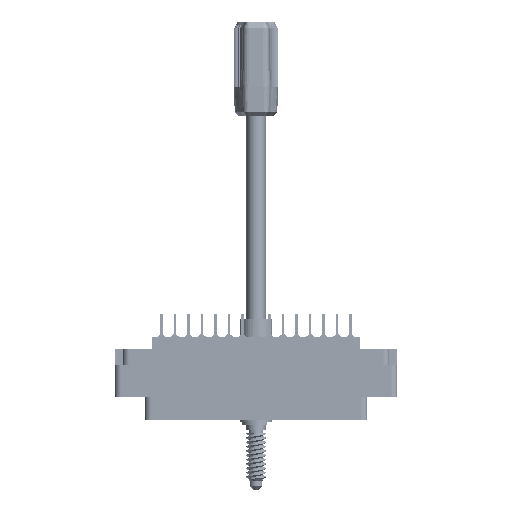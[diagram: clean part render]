
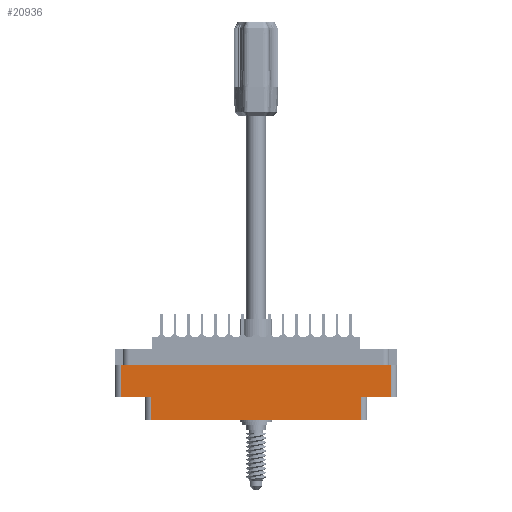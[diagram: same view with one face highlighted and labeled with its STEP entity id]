
A CAD part, front view. The second image highlights one B-rep face of the part: STEP entity #20936.
In plain terms, the highlighted planar face has unit normal (0, -1, 0).
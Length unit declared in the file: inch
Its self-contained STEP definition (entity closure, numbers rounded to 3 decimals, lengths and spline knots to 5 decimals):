
#2344 = LINE ( 'NONE', #57740, #59370 ) ;
#3108 = VERTEX_POINT ( 'NONE', #76428 ) ;
#3857 = CARTESIAN_POINT ( 'NONE',  ( -1.359, -0.617, -0.798 ) ) ;
#4095 = CARTESIAN_POINT ( 'NONE',  ( -1.297, -0.617, -0.578 ) ) ;
#4109 = ORIENTED_EDGE ( 'NONE', *, *, #5553, .F. ) ;
#5553 = EDGE_CURVE ( 'NONE', #71002, #6248, #46296, .T. ) ;
#6248 = VERTEX_POINT ( 'NONE', #72584 ) ;
#6738 = VERTEX_POINT ( 'NONE', #8412 ) ;
#7164 = VERTEX_POINT ( 'NONE', #36387 ) ;
#8156 = ORIENTED_EDGE ( 'NONE', *, *, #20515, .T. ) ;
#8412 = CARTESIAN_POINT ( 'NONE',  ( -1.006, -0.617, -0.798 ) ) ;
#8616 = VERTEX_POINT ( 'NONE', #9240 ) ;
#9240 = CARTESIAN_POINT ( 'NONE',  ( -1.006, -0.617, -0.578 ) ) ;
#9467 = EDGE_CURVE ( 'NONE', #8616, #6738, #44983, .T. ) ;
#11012 = DIRECTION ( 'NONE',  ( 1., 0., 0. ) ) ;
#11029 = EDGE_CURVE ( 'NONE', #15318, #8616, #67123, .T. ) ;
#11139 = VECTOR ( 'NONE', #11012, 39.37008 ) ;
#14254 = EDGE_CURVE ( 'NONE', #6738, #7164, #2344, .T. ) ;
#15318 = VERTEX_POINT ( 'NONE', #4095 ) ;
#16478 = VECTOR ( 'NONE', #76338, 39.37008 ) ;
#18670 = CARTESIAN_POINT ( 'NONE',  ( 0., -0.617, -0.578 ) ) ;
#20515 = EDGE_CURVE ( 'NONE', #73805, #6248, #29025, .T. ) ;
#20936 = ADVANCED_FACE ( 'NONE', ( #48536 ), #24695, .T. ) ;
#21580 = CARTESIAN_POINT ( 'NONE',  ( -1.297, -0.617, -0.274 ) ) ;
#22861 = VECTOR ( 'NONE', #69474, 39.37008 ) ;
#24181 = ORIENTED_EDGE ( 'NONE', *, *, #29107, .F. ) ;
#24695 = PLANE ( 'NONE',  #72409 ) ;
#27738 = VECTOR ( 'NONE', #43543, 39.37008 ) ;
#29025 = LINE ( 'NONE', #62917, #22861 ) ;
#29107 = EDGE_CURVE ( 'NONE', #73805, #3108, #46611, .T. ) ;
#33746 = VECTOR ( 'NONE', #73621, 39.37008 ) ;
#36387 = CARTESIAN_POINT ( 'NONE',  ( 1.006, -0.617, -0.798 ) ) ;
#40005 = CARTESIAN_POINT ( 'NONE',  ( 0., -0.617, -0.274 ) ) ;
#40522 = VECTOR ( 'NONE', #76292, 39.37008 ) ;
#42891 = DIRECTION ( 'NONE',  ( 0., 0., -1. ) ) ;
#42982 = CARTESIAN_POINT ( 'NONE',  ( -1.297, -0.617, -0.798 ) ) ;
#43543 = DIRECTION ( 'NONE',  ( 0., 0., -1. ) ) ;
#44983 = LINE ( 'NONE', #84278, #16478 ) ;
#46296 = LINE ( 'NONE', #40005, #67701 ) ;
#46611 = LINE ( 'NONE', #56333, #40522 ) ;
#46760 = DIRECTION ( 'NONE',  ( 1., 0., 0. ) ) ;
#46912 = LINE ( 'NONE', #47671, #33746 ) ;
#47557 = EDGE_LOOP ( 'NONE', ( #48746, #52142, #61343, #48615, #24181, #8156, #4109, #60714 ) ) ;
#47671 = CARTESIAN_POINT ( 'NONE',  ( 1.006, -0.617, -0.578 ) ) ;
#48536 = FACE_OUTER_BOUND ( 'NONE', #47557, .T. ) ;
#48615 = ORIENTED_EDGE ( 'NONE', *, *, #58975, .T. ) ;
#48746 = ORIENTED_EDGE ( 'NONE', *, *, #11029, .T. ) ;
#52142 = ORIENTED_EDGE ( 'NONE', *, *, #9467, .T. ) ;
#56333 = CARTESIAN_POINT ( 'NONE',  ( 0., -0.617, -0.578 ) ) ;
#56834 = CARTESIAN_POINT ( 'NONE',  ( 1.297, -0.617, -0.578 ) ) ;
#57740 = CARTESIAN_POINT ( 'NONE',  ( -1.359, -0.617, -0.798 ) ) ;
#58975 = EDGE_CURVE ( 'NONE', #7164, #3108, #46912, .T. ) ;
#59370 = VECTOR ( 'NONE', #63762, 39.37008 ) ;
#60714 = ORIENTED_EDGE ( 'NONE', *, *, #69272, .T. ) ;
#61343 = ORIENTED_EDGE ( 'NONE', *, *, #14254, .T. ) ;
#62515 = DIRECTION ( 'NONE',  ( 0., -1., 0. ) ) ;
#62917 = CARTESIAN_POINT ( 'NONE',  ( 1.297, -0.617, -0.798 ) ) ;
#63762 = DIRECTION ( 'NONE',  ( 1., 0., 0. ) ) ;
#67123 = LINE ( 'NONE', #18670, #11139 ) ;
#67701 = VECTOR ( 'NONE', #46760, 39.37008 ) ;
#69272 = EDGE_CURVE ( 'NONE', #71002, #15318, #70511, .T. ) ;
#69474 = DIRECTION ( 'NONE',  ( 0., 0., 1. ) ) ;
#70511 = LINE ( 'NONE', #42982, #27738 ) ;
#71002 = VERTEX_POINT ( 'NONE', #21580 ) ;
#72409 = AXIS2_PLACEMENT_3D ( 'NONE', #3857, #62515, #42891 ) ;
#72584 = CARTESIAN_POINT ( 'NONE',  ( 1.297, -0.617, -0.274 ) ) ;
#73621 = DIRECTION ( 'NONE',  ( 0., 0., 1. ) ) ;
#73805 = VERTEX_POINT ( 'NONE', #56834 ) ;
#76292 = DIRECTION ( 'NONE',  ( -1., 0., 0. ) ) ;
#76338 = DIRECTION ( 'NONE',  ( 0., 0., -1. ) ) ;
#76428 = CARTESIAN_POINT ( 'NONE',  ( 1.006, -0.617, -0.578 ) ) ;
#84278 = CARTESIAN_POINT ( 'NONE',  ( -1.006, -0.617, -0.798 ) ) ;
